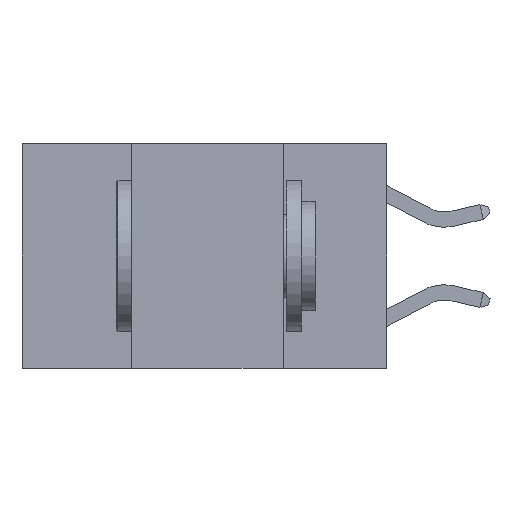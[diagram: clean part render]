
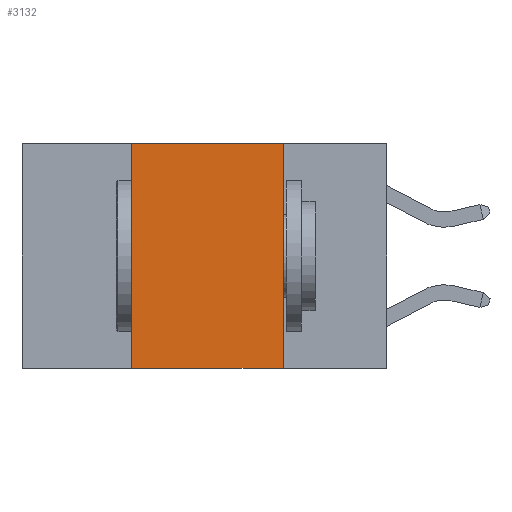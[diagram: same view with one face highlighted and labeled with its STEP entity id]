
A CAD part, left-side view. The second image highlights one B-rep face of the part: STEP entity #3132.
In plain terms, the highlighted planar face has unit normal (-1, 0, 0).
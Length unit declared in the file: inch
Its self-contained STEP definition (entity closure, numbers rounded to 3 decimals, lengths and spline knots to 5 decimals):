
#527 = VERTEX_POINT ( 'NONE', #6390 ) ;
#580 = CARTESIAN_POINT ( 'NONE',  ( 0., 0.6, -0.37 ) ) ;
#1040 = VECTOR ( 'NONE', #10403, 39.37008 ) ;
#1521 = VERTEX_POINT ( 'NONE', #13457 ) ;
#3132 = ADVANCED_FACE ( 'NONE', ( #9394 ), #3406, .F. ) ;
#3145 = VERTEX_POINT ( 'NONE', #3509 ) ;
#3406 = PLANE ( 'NONE',  #10205 ) ;
#3509 = CARTESIAN_POINT ( 'NONE',  ( 0., 0.42, 0. ) ) ;
#3577 = EDGE_CURVE ( 'NONE', #10571, #527, #16505, .T. ) ;
#5907 = VECTOR ( 'NONE', #11611, 39.37008 ) ;
#6379 = CARTESIAN_POINT ( 'NONE',  ( 0., 0.42, 0. ) ) ;
#6390 = CARTESIAN_POINT ( 'NONE',  ( 0., 0.17, -0.37 ) ) ;
#7125 = VECTOR ( 'NONE', #14802, 39.37008 ) ;
#7177 = VECTOR ( 'NONE', #16884, 39.37008 ) ;
#7559 = CARTESIAN_POINT ( 'NONE',  ( 0., 0.42, -0.37 ) ) ;
#9078 = LINE ( 'NONE', #6379, #1040 ) ;
#9394 = FACE_OUTER_BOUND ( 'NONE', #11812, .T. ) ;
#9679 = EDGE_CURVE ( 'NONE', #10571, #3145, #9078, .T. ) ;
#10127 = ORIENTED_EDGE ( 'NONE', *, *, #14021, .F. ) ;
#10133 = CARTESIAN_POINT ( 'NONE',  ( 0., 0.6, 0. ) ) ;
#10205 = AXIS2_PLACEMENT_3D ( 'NONE', #16331, #14922, #15104 ) ;
#10403 = DIRECTION ( 'NONE',  ( 0., 0., 1. ) ) ;
#10571 = VERTEX_POINT ( 'NONE', #7559 ) ;
#11611 = DIRECTION ( 'NONE',  ( 0., -1., 0. ) ) ;
#11812 = EDGE_LOOP ( 'NONE', ( #13176, #10127, #12990, #15541 ) ) ;
#12990 = ORIENTED_EDGE ( 'NONE', *, *, #9679, .F. ) ;
#13176 = ORIENTED_EDGE ( 'NONE', *, *, #16829, .F. ) ;
#13457 = CARTESIAN_POINT ( 'NONE',  ( 0., 0.17, 0. ) ) ;
#14021 = EDGE_CURVE ( 'NONE', #3145, #1521, #17522, .T. ) ;
#14059 = LINE ( 'NONE', #16981, #7177 ) ;
#14802 = DIRECTION ( 'NONE',  ( 0., -1., 0. ) ) ;
#14922 = DIRECTION ( 'NONE',  ( 1., 0., 0. ) ) ;
#15104 = DIRECTION ( 'NONE',  ( 0., 0., -1. ) ) ;
#15541 = ORIENTED_EDGE ( 'NONE', *, *, #3577, .T. ) ;
#16331 = CARTESIAN_POINT ( 'NONE',  ( 0., 0.6, 0. ) ) ;
#16505 = LINE ( 'NONE', #580, #7125 ) ;
#16829 = EDGE_CURVE ( 'NONE', #1521, #527, #14059, .T. ) ;
#16884 = DIRECTION ( 'NONE',  ( 0., 0., -1. ) ) ;
#16981 = CARTESIAN_POINT ( 'NONE',  ( 0., 0.17, 0. ) ) ;
#17522 = LINE ( 'NONE', #10133, #5907 ) ;
